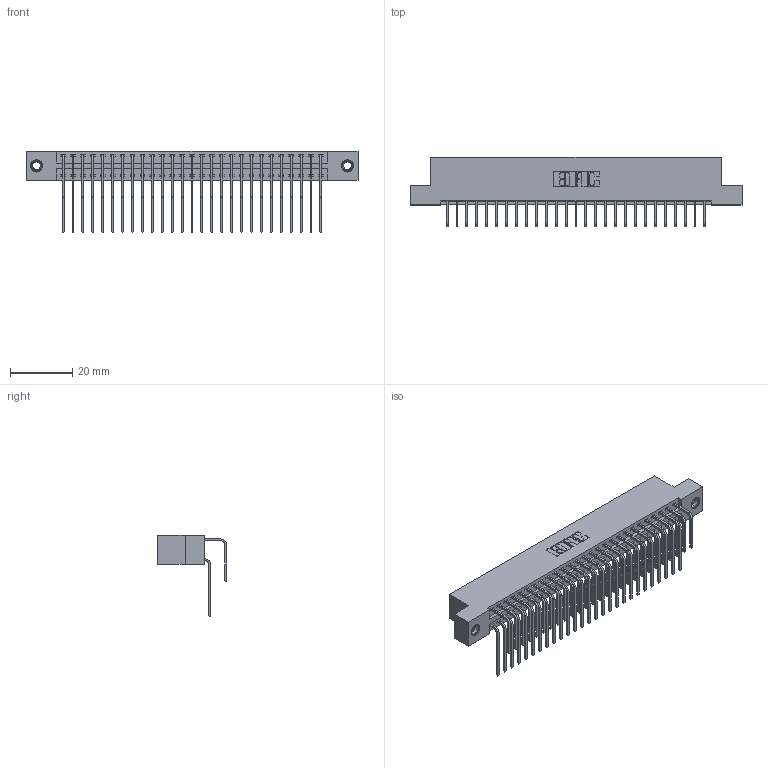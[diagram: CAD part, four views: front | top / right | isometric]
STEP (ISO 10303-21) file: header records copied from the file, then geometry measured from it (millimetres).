
FILE_DESCRIPTION (( 'STEP AP203' ), '1' );
FILE_NAME ('346-054-558-207.STEP', '2022-05-21T04:12:42', ( '' ), ( '' ), 'SwSTEP 2.0', 'SolidWorks 2020', '' );
FILE_SCHEMA (( 'CONFIG_CONTROL_DESIGN' ));
Length unit declared in the file: inch
Products named in the file (5): 345-292-001_558 Tail - 2; 346 Part_Flush Mounting Lugs - 0.156 Dia-TI; 346-054-558-207; 345-292-001_558 559 Tail - 1; 345-250-001_345-250-005-103
Assembly tree (57 placements, depth 2):
  346-054-558-207
    346 Part_Flush Mounting Lugs - 0.156 Dia-TI
    345-292-001_558 559 Tail - 1  x27
    345-292-001_558 Tail - 2  x27
    345-250-001_345-250-005-103  x2
Bounding box: 106.3 x 22.16 x 26.16 mm (x, y, z)
Volume: 10547 mm3; surface area: 15789.9 mm2
Topology: 57 solids, 57 shells, 3098 faces, 9159 edges, 6026 vertices
Faces by surface type: plane 2106, cylinder 976, cone 12, torus 4
Entity records: 22610 total; most frequent: CARTESIAN_POINT 3782, ORIENTED_EDGE 3658, DIRECTION 3383, EDGE_CURVE 1829, LINE 1529, VECTOR 1529, VERTEX_POINT 1212, AXIS2_PLACEMENT_3D 927
